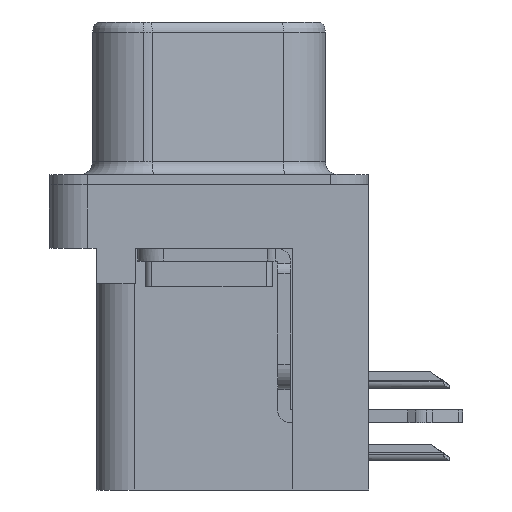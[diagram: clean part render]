
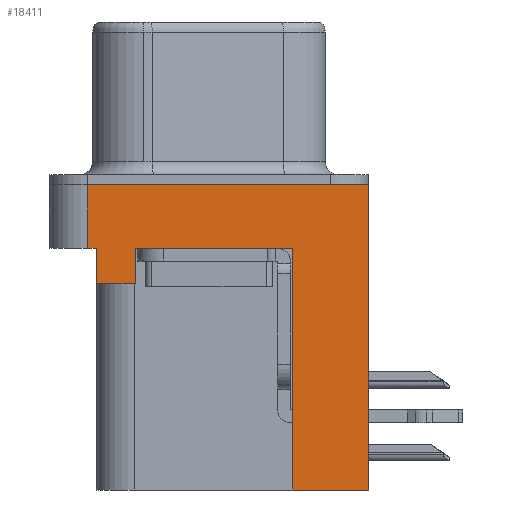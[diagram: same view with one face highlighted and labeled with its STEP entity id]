
A CAD part, left-side view. The second image highlights one B-rep face of the part: STEP entity #18411.
In plain terms, the highlighted planar face has unit normal (-1, 0, 0).
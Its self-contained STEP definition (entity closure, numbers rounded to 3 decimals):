
#12 = EDGE_CURVE ( 'NONE', #10169, #16500, #10117, .T. ) ;
#708 = CARTESIAN_POINT ( 'NONE',  ( -3., 4.425, -2.5 ) ) ;
#727 = DIRECTION ( 'NONE',  ( 0., 1., 0. ) ) ;
#858 = DIRECTION ( 'NONE',  ( 0., 1., 0. ) ) ;
#1251 = DIRECTION ( 'NONE',  ( 0., 0., 1. ) ) ;
#1492 = CARTESIAN_POINT ( 'NONE',  ( -3., 4.425, -3.9 ) ) ;
#2074 = LINE ( 'NONE', #16623, #12297 ) ;
#2136 = EDGE_CURVE ( 'NONE', #9854, #21990, #16387, .T. ) ;
#2549 = CARTESIAN_POINT ( 'NONE',  ( -3., 2.895, -3.9 ) ) ;
#2587 = CARTESIAN_POINT ( 'NONE',  ( -3., 2.895, -2.5 ) ) ;
#2954 = VECTOR ( 'NONE', #858, 1000. ) ;
#2993 = EDGE_CURVE ( 'NONE', #9933, #22423, #22503, .T. ) ;
#3093 = VECTOR ( 'NONE', #5839, 1000. ) ;
#3315 = CARTESIAN_POINT ( 'NONE',  ( -3., 4.425, -3.9 ) ) ;
#4420 = DIRECTION ( 'NONE',  ( 0., 0., 1. ) ) ;
#5219 = ORIENTED_EDGE ( 'NONE', *, *, #10946, .F. ) ;
#5357 = LINE ( 'NONE', #14266, #18709 ) ;
#5373 = VECTOR ( 'NONE', #22767, 1000. ) ;
#5420 = DIRECTION ( 'NONE',  ( 0., -1., 0. ) ) ;
#5600 = EDGE_CURVE ( 'NONE', #15705, #21990, #14823, .T. ) ;
#5778 = CARTESIAN_POINT ( 'NONE',  ( -3., 4.775, 0. ) ) ;
#5819 = CARTESIAN_POINT ( 'NONE',  ( -3., 2.895, -3.9 ) ) ;
#5833 = EDGE_CURVE ( 'NONE', #16637, #22423, #2074, .T. ) ;
#5839 = DIRECTION ( 'NONE',  ( 0., -1., 0. ) ) ;
#6340 = CARTESIAN_POINT ( 'NONE',  ( -3., 4.775, -2.5 ) ) ;
#8016 = ORIENTED_EDGE ( 'NONE', *, *, #18590, .F. ) ;
#8082 = ORIENTED_EDGE ( 'NONE', *, *, #5600, .T. ) ;
#8687 = VECTOR ( 'NONE', #727, 1000. ) ;
#9854 = VERTEX_POINT ( 'NONE', #5778 ) ;
#9933 = VERTEX_POINT ( 'NONE', #3315 ) ;
#10117 = LINE ( 'NONE', #5819, #13767 ) ;
#10169 = VERTEX_POINT ( 'NONE', #2549 ) ;
#10267 = ORIENTED_EDGE ( 'NONE', *, *, #12, .T. ) ;
#10402 = EDGE_CURVE ( 'NONE', #16845, #17810, #14824, .T. ) ;
#10524 = VECTOR ( 'NONE', #4420, 1000. ) ;
#10946 = EDGE_CURVE ( 'NONE', #10169, #9933, #19784, .T. ) ;
#11225 = CARTESIAN_POINT ( 'NONE',  ( -3., -6.275, -2.5 ) ) ;
#12223 = PLANE ( 'NONE',  #13153 ) ;
#12297 = VECTOR ( 'NONE', #18495, 1000. ) ;
#12379 = CARTESIAN_POINT ( 'NONE',  ( -3., -6.275, -2.5 ) ) ;
#12759 = DIRECTION ( 'NONE',  ( -1., 0., 0. ) ) ;
#13153 = AXIS2_PLACEMENT_3D ( 'NONE', #12379, #12759, #16320 ) ;
#13767 = VECTOR ( 'NONE', #21819, 1000. ) ;
#14263 = CARTESIAN_POINT ( 'NONE',  ( -3., 4.775, -2.5 ) ) ;
#14266 = CARTESIAN_POINT ( 'NONE',  ( -3., -6.275, -2.5 ) ) ;
#14518 = DIRECTION ( 'NONE',  ( 0., 0., 1. ) ) ;
#14541 = CARTESIAN_POINT ( 'NONE',  ( -3., -3.295, -12. ) ) ;
#14693 = CARTESIAN_POINT ( 'NONE',  ( -3., -6.275, 0. ) ) ;
#14801 = ORIENTED_EDGE ( 'NONE', *, *, #5833, .T. ) ;
#14823 = LINE ( 'NONE', #11225, #15929 ) ;
#14824 = LINE ( 'NONE', #15476, #5373 ) ;
#14952 = CARTESIAN_POINT ( 'NONE',  ( -3., -3.295, -12. ) ) ;
#15281 = LINE ( 'NONE', #6340, #10524 ) ;
#15476 = CARTESIAN_POINT ( 'NONE',  ( -3., -3.295, -12. ) ) ;
#15705 = VERTEX_POINT ( 'NONE', #20778 ) ;
#15922 = EDGE_CURVE ( 'NONE', #16500, #17810, #5357, .T. ) ;
#15929 = VECTOR ( 'NONE', #14518, 1000. ) ;
#16320 = DIRECTION ( 'NONE',  ( 0., 0., 1. ) ) ;
#16387 = LINE ( 'NONE', #14693, #3093 ) ;
#16500 = VERTEX_POINT ( 'NONE', #2587 ) ;
#16623 = CARTESIAN_POINT ( 'NONE',  ( -3., -6.275, -2.5 ) ) ;
#16637 = VERTEX_POINT ( 'NONE', #14263 ) ;
#16845 = VERTEX_POINT ( 'NONE', #14541 ) ;
#17505 = ORIENTED_EDGE ( 'NONE', *, *, #22498, .F. ) ;
#17810 = VERTEX_POINT ( 'NONE', #21045 ) ;
#18411 = ADVANCED_FACE ( 'NONE', ( #20290 ), #12223, .T. ) ;
#18495 = DIRECTION ( 'NONE',  ( 0., -1., 0. ) ) ;
#18590 = EDGE_CURVE ( 'NONE', #16637, #9854, #15281, .T. ) ;
#18605 = VECTOR ( 'NONE', #1251, 1000. ) ;
#18709 = VECTOR ( 'NONE', #5420, 1000. ) ;
#19294 = ORIENTED_EDGE ( 'NONE', *, *, #15922, .T. ) ;
#19784 = LINE ( 'NONE', #20320, #8687 ) ;
#20153 = LINE ( 'NONE', #14952, #2954 ) ;
#20290 = FACE_OUTER_BOUND ( 'NONE', #22453, .T. ) ;
#20320 = CARTESIAN_POINT ( 'NONE',  ( -3., 4.425, -3.9 ) ) ;
#20635 = CARTESIAN_POINT ( 'NONE',  ( -3., -6.275, 0. ) ) ;
#20667 = ORIENTED_EDGE ( 'NONE', *, *, #10402, .F. ) ;
#20778 = CARTESIAN_POINT ( 'NONE',  ( -3., -6.275, -12. ) ) ;
#21045 = CARTESIAN_POINT ( 'NONE',  ( -3., -3.295, -2.5 ) ) ;
#21490 = ORIENTED_EDGE ( 'NONE', *, *, #2993, .F. ) ;
#21819 = DIRECTION ( 'NONE',  ( 0., 0., 1. ) ) ;
#21990 = VERTEX_POINT ( 'NONE', #20635 ) ;
#22423 = VERTEX_POINT ( 'NONE', #708 ) ;
#22453 = EDGE_LOOP ( 'NONE', ( #22825, #8016, #14801, #21490, #5219, #10267, #19294, #20667, #17505, #8082 ) ) ;
#22498 = EDGE_CURVE ( 'NONE', #15705, #16845, #20153, .T. ) ;
#22503 = LINE ( 'NONE', #1492, #18605 ) ;
#22767 = DIRECTION ( 'NONE',  ( 0., 0., 1. ) ) ;
#22825 = ORIENTED_EDGE ( 'NONE', *, *, #2136, .F. ) ;
